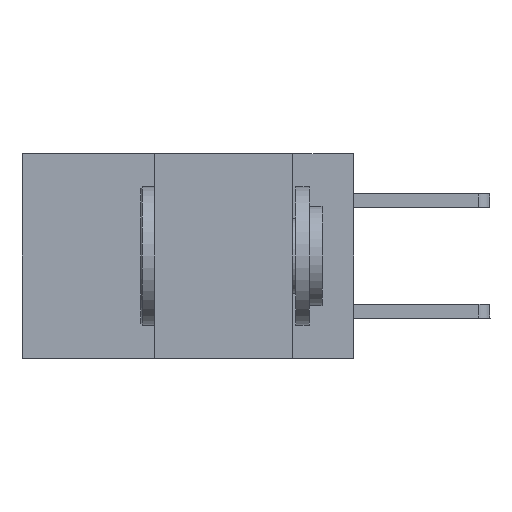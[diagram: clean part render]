
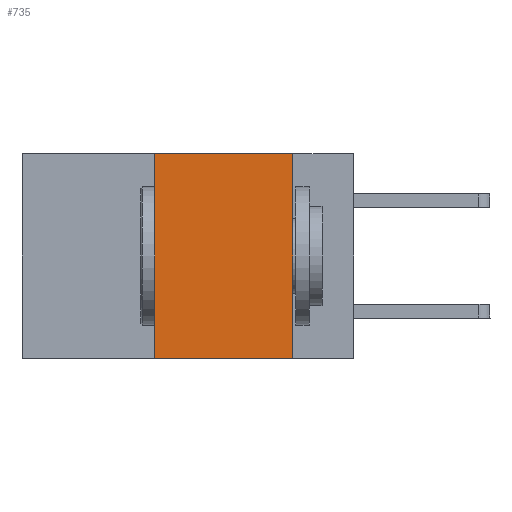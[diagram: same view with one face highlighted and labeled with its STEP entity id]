
A CAD part, left-side view. The second image highlights one B-rep face of the part: STEP entity #735.
In plain terms, the highlighted planar face has unit normal (-1, 0, 0).
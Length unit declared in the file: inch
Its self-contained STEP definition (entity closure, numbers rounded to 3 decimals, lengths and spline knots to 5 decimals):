
#29 = PLANE ( 'NONE',  #3744 ) ;
#582 = VERTEX_POINT ( 'NONE', #5617 ) ;
#609 = VECTOR ( 'NONE', #4569, 39.37008 ) ;
#735 = ADVANCED_FACE ( 'NONE', ( #3964 ), #29, .F. ) ;
#774 = VERTEX_POINT ( 'NONE', #8504 ) ;
#1121 = CARTESIAN_POINT ( 'NONE',  ( 0., 0.11, 0. ) ) ;
#1288 = VERTEX_POINT ( 'NONE', #11595 ) ;
#2066 = LINE ( 'NONE', #1121, #6838 ) ;
#2132 = EDGE_CURVE ( 'NONE', #582, #5329, #2066, .T. ) ;
#2327 = CARTESIAN_POINT ( 'NONE',  ( 0., 0.36, 0. ) ) ;
#3076 = CARTESIAN_POINT ( 'NONE',  ( 0., 0.6, 0. ) ) ;
#3248 = LINE ( 'NONE', #8407, #10737 ) ;
#3744 = AXIS2_PLACEMENT_3D ( 'NONE', #3076, #6206, #6078 ) ;
#3964 = FACE_OUTER_BOUND ( 'NONE', #6871, .T. ) ;
#4385 = EDGE_CURVE ( 'NONE', #774, #5329, #8784, .T. ) ;
#4569 = DIRECTION ( 'NONE',  ( 0., 0., 1. ) ) ;
#4905 = VECTOR ( 'NONE', #12978, 39.37008 ) ;
#5023 = ORIENTED_EDGE ( 'NONE', *, *, #11171, .F. ) ;
#5329 = VERTEX_POINT ( 'NONE', #6222 ) ;
#5617 = CARTESIAN_POINT ( 'NONE',  ( 0., 0.11, 0. ) ) ;
#6078 = DIRECTION ( 'NONE',  ( 0., 0., -1. ) ) ;
#6206 = DIRECTION ( 'NONE',  ( 1., 0., 0. ) ) ;
#6222 = CARTESIAN_POINT ( 'NONE',  ( 0., 0.11, -0.37 ) ) ;
#6838 = VECTOR ( 'NONE', #13535, 39.37008 ) ;
#6871 = EDGE_LOOP ( 'NONE', ( #9311, #12530, #5023, #13363 ) ) ;
#7814 = CARTESIAN_POINT ( 'NONE',  ( 0., 0.6, -0.37 ) ) ;
#8407 = CARTESIAN_POINT ( 'NONE',  ( 0., 0.6, 0. ) ) ;
#8504 = CARTESIAN_POINT ( 'NONE',  ( 0., 0.36, -0.37 ) ) ;
#8562 = LINE ( 'NONE', #2327, #609 ) ;
#8784 = LINE ( 'NONE', #7814, #4905 ) ;
#9311 = ORIENTED_EDGE ( 'NONE', *, *, #2132, .F. ) ;
#9829 = EDGE_CURVE ( 'NONE', #1288, #582, #3248, .T. ) ;
#10737 = VECTOR ( 'NONE', #12606, 39.37008 ) ;
#11171 = EDGE_CURVE ( 'NONE', #774, #1288, #8562, .T. ) ;
#11595 = CARTESIAN_POINT ( 'NONE',  ( 0., 0.36, 0. ) ) ;
#12530 = ORIENTED_EDGE ( 'NONE', *, *, #9829, .F. ) ;
#12606 = DIRECTION ( 'NONE',  ( 0., -1., 0. ) ) ;
#12978 = DIRECTION ( 'NONE',  ( 0., -1., 0. ) ) ;
#13363 = ORIENTED_EDGE ( 'NONE', *, *, #4385, .T. ) ;
#13535 = DIRECTION ( 'NONE',  ( 0., 0., -1. ) ) ;
